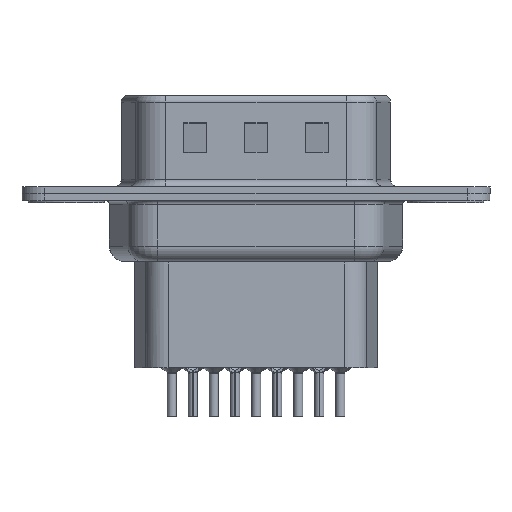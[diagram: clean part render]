
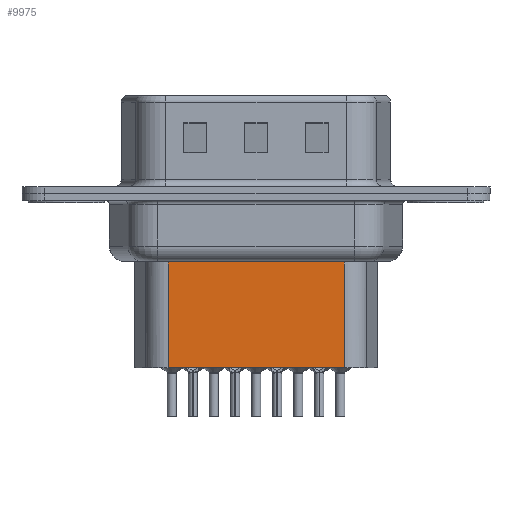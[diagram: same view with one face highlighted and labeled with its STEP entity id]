
A CAD part, front view. The second image highlights one B-rep face of the part: STEP entity #9975.
In plain terms, the highlighted planar face has unit normal (0, -1, 0).
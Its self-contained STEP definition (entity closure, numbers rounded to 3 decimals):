
#23 = DIRECTION ( 'NONE',  ( 0., -1., 0. ) ) ;
#465 = VERTEX_POINT ( 'NONE', #4302 ) ;
#605 = CARTESIAN_POINT ( 'NONE',  ( 18.294, -3.5, -3.1 ) ) ;
#661 = DIRECTION ( 'NONE',  ( -1., 0., 0. ) ) ;
#1511 = ORIENTED_EDGE ( 'NONE', *, *, #4427, .F. ) ;
#1607 = ORIENTED_EDGE ( 'NONE', *, *, #16589, .F. ) ;
#2424 = VERTEX_POINT ( 'NONE', #3712 ) ;
#2432 = LINE ( 'NONE', #605, #5471 ) ;
#2692 = ORIENTED_EDGE ( 'NONE', *, *, #8165, .T. ) ;
#2967 = VERTEX_POINT ( 'NONE', #15015 ) ;
#3712 = CARTESIAN_POINT ( 'NONE',  ( 18.294, -3.5, -4.097 ) ) ;
#3995 = FACE_OUTER_BOUND ( 'NONE', #4538, .T. ) ;
#4302 = CARTESIAN_POINT ( 'NONE',  ( 6.706, -3.5, -4.097 ) ) ;
#4427 = EDGE_CURVE ( 'NONE', #2967, #9345, #7644, .T. ) ;
#4538 = EDGE_LOOP ( 'NONE', ( #1607, #2692, #10699, #1511 ) ) ;
#5471 = VECTOR ( 'NONE', #13545, 1000. ) ;
#5619 = DIRECTION ( 'NONE',  ( 0., 0., -1. ) ) ;
#6171 = VECTOR ( 'NONE', #5619, 1000. ) ;
#6927 = CARTESIAN_POINT ( 'NONE',  ( 6.706, -3.5, -3.1 ) ) ;
#7644 = LINE ( 'NONE', #16173, #14127 ) ;
#7773 = CARTESIAN_POINT ( 'NONE',  ( 6.706, -3.5, -3.1 ) ) ;
#8080 = VECTOR ( 'NONE', #12842, 1000. ) ;
#8165 = EDGE_CURVE ( 'NONE', #2424, #465, #11538, .T. ) ;
#9007 = CARTESIAN_POINT ( 'NONE',  ( 6.459, -3.5, -4.097 ) ) ;
#9077 = DIRECTION ( 'NONE',  ( 1., 0., 0. ) ) ;
#9345 = VERTEX_POINT ( 'NONE', #13690 ) ;
#9598 = LINE ( 'NONE', #6927, #6171 ) ;
#9975 = ADVANCED_FACE ( 'NONE', ( #3995 ), #15547, .T. ) ;
#10179 = EDGE_CURVE ( 'NONE', #465, #9345, #9598, .T. ) ;
#10699 = ORIENTED_EDGE ( 'NONE', *, *, #10179, .T. ) ;
#11538 = LINE ( 'NONE', #9007, #8080 ) ;
#12842 = DIRECTION ( 'NONE',  ( -1., 0., 0. ) ) ;
#13545 = DIRECTION ( 'NONE',  ( 0., 0., -1. ) ) ;
#13690 = CARTESIAN_POINT ( 'NONE',  ( 6.706, -3.5, -11.45 ) ) ;
#13758 = AXIS2_PLACEMENT_3D ( 'NONE', #7773, #23, #9077 ) ;
#14127 = VECTOR ( 'NONE', #661, 1000. ) ;
#15015 = CARTESIAN_POINT ( 'NONE',  ( 18.294, -3.5, -11.45 ) ) ;
#15547 = PLANE ( 'NONE',  #13758 ) ;
#16173 = CARTESIAN_POINT ( 'NONE',  ( 6.706, -3.5, -11.45 ) ) ;
#16589 = EDGE_CURVE ( 'NONE', #2424, #2967, #2432, .T. ) ;
